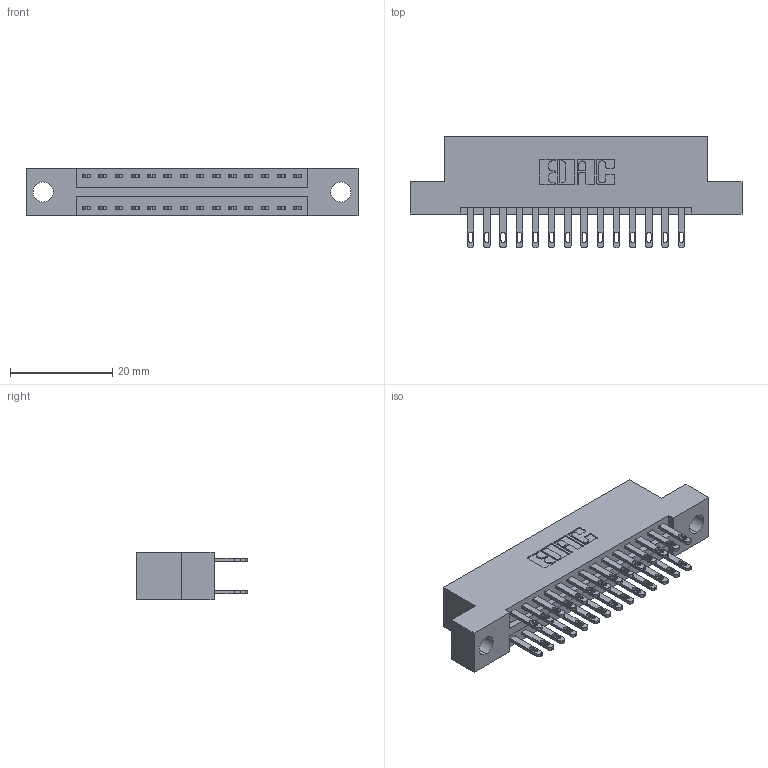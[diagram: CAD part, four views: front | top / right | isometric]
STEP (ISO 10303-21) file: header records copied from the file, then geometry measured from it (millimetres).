
FILE_DESCRIPTION (( 'STEP AP203' ), '1' );
FILE_NAME ('346-028-500-204.STEP', '2022-05-19T03:20:28', ( '' ), ( '' ), 'SwSTEP 2.0', 'SolidWorks 2020', '' );
FILE_SCHEMA (( 'CONFIG_CONTROL_DESIGN' ));
Length unit declared in the file: inch
Products named in the file (3): 346-028-500-204; 346 Part_Flush Mounting Lugs - 0.156 Dia-TH; 345-292-001_345-293-100
Assembly tree (29 placements, depth 2):
  346-028-500-204
    346 Part_Flush Mounting Lugs - 0.156 Dia-TH
    345-292-001_345-293-100  x28
Bounding box: 65.02 x 21.84 x 9.4 mm (x, y, z)
Volume: 6102.8 mm3; surface area: 8089.6 mm2
Topology: 29 solids, 29 shells, 1480 faces, 4481 edges, 2986 vertices
Faces by surface type: plane 902, cylinder 578
Entity records: 13255 total; most frequent: CARTESIAN_POINT 2226, ORIENTED_EDGE 2158, DIRECTION 2015, EDGE_CURVE 1079, VECTOR 887, LINE 887, VERTEX_POINT 718, AXIS2_PLACEMENT_3D 564
